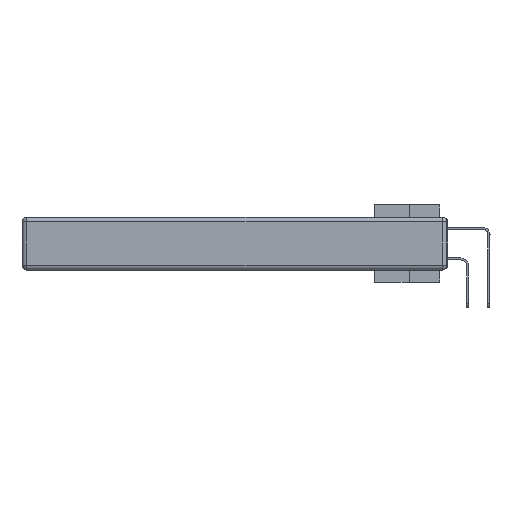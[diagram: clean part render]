
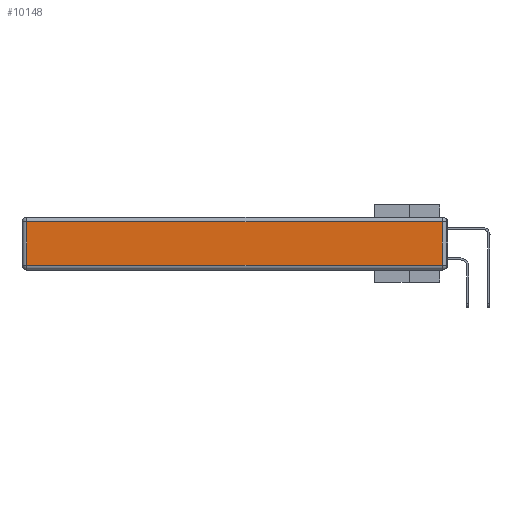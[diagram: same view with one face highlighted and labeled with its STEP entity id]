
A CAD part, left-side view. The second image highlights one B-rep face of the part: STEP entity #10148.
In plain terms, the highlighted planar face has unit normal (-1, 0, 0).
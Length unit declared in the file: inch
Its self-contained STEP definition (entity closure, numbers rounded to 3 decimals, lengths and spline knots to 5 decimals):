
#934 = CARTESIAN_POINT ( 'NONE',  ( 0., 0., -0.313 ) ) ;
#3969 = DIRECTION ( 'NONE',  ( 0., -1., 0. ) ) ;
#4216 = CARTESIAN_POINT ( 'NONE',  ( 0., 0.03, -0.03 ) ) ;
#4955 = CARTESIAN_POINT ( 'NONE',  ( 0., 2.75, -0.03 ) ) ;
#6396 = VERTEX_POINT ( 'NONE', #4216 ) ;
#8460 = DIRECTION ( 'NONE',  ( -1., 0., 0. ) ) ;
#10148 = ADVANCED_FACE ( 'NONE', ( #16708 ), #28030, .T. ) ;
#10418 = LINE ( 'NONE', #26587, #21233 ) ;
#10509 = LINE ( 'NONE', #4955, #15455 ) ;
#11326 = DIRECTION ( 'NONE',  ( 0., 0., 1. ) ) ;
#12056 = CARTESIAN_POINT ( 'NONE',  ( 0., 2.72, -0.03 ) ) ;
#12154 = EDGE_CURVE ( 'NONE', #35236, #13457, #34954, .T. ) ;
#12351 = CARTESIAN_POINT ( 'NONE',  ( 0., 2.72, -0.343 ) ) ;
#12930 = DIRECTION ( 'NONE',  ( 0., 0., 1. ) ) ;
#13457 = VERTEX_POINT ( 'NONE', #24190 ) ;
#13768 = EDGE_LOOP ( 'NONE', ( #24641, #33380, #30348, #31872 ) ) ;
#15455 = VECTOR ( 'NONE', #32051, 39.37008 ) ;
#16708 = FACE_OUTER_BOUND ( 'NONE', #13768, .T. ) ;
#18295 = VECTOR ( 'NONE', #20587, 39.37008 ) ;
#19966 = VECTOR ( 'NONE', #3969, 39.37008 ) ;
#20587 = DIRECTION ( 'NONE',  ( 0., 0., -1. ) ) ;
#21233 = VECTOR ( 'NONE', #12930, 39.37008 ) ;
#21965 = EDGE_CURVE ( 'NONE', #6396, #35236, #10509, .T. ) ;
#22079 = CARTESIAN_POINT ( 'NONE',  ( 0., 0., -0.343 ) ) ;
#22784 = EDGE_CURVE ( 'NONE', #23366, #6396, #10418, .T. ) ;
#23329 = LINE ( 'NONE', #934, #19966 ) ;
#23366 = VERTEX_POINT ( 'NONE', #30482 ) ;
#23901 = AXIS2_PLACEMENT_3D ( 'NONE', #22079, #8460, #11326 ) ;
#24190 = CARTESIAN_POINT ( 'NONE',  ( 0., 2.72, -0.313 ) ) ;
#24641 = ORIENTED_EDGE ( 'NONE', *, *, #32120, .T. ) ;
#26587 = CARTESIAN_POINT ( 'NONE',  ( 0., 0.03, -0.343 ) ) ;
#28030 = PLANE ( 'NONE',  #23901 ) ;
#30348 = ORIENTED_EDGE ( 'NONE', *, *, #21965, .T. ) ;
#30482 = CARTESIAN_POINT ( 'NONE',  ( 0., 0.03, -0.313 ) ) ;
#31872 = ORIENTED_EDGE ( 'NONE', *, *, #12154, .T. ) ;
#32051 = DIRECTION ( 'NONE',  ( 0., 1., 0. ) ) ;
#32120 = EDGE_CURVE ( 'NONE', #13457, #23366, #23329, .T. ) ;
#33380 = ORIENTED_EDGE ( 'NONE', *, *, #22784, .T. ) ;
#34954 = LINE ( 'NONE', #12351, #18295 ) ;
#35236 = VERTEX_POINT ( 'NONE', #12056 ) ;
